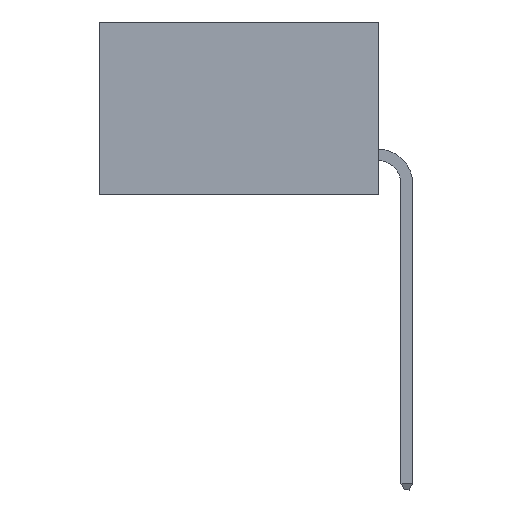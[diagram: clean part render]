
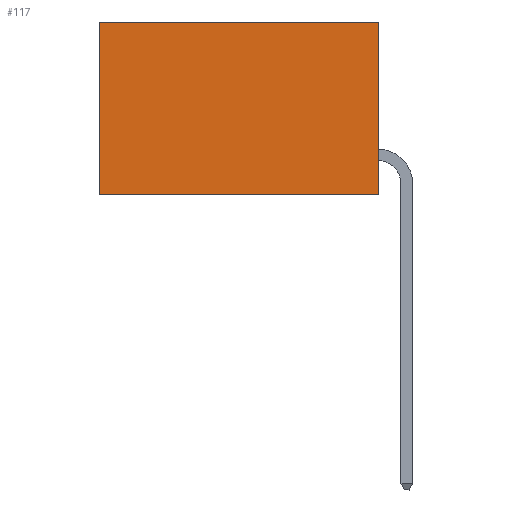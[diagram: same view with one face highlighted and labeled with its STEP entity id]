
A CAD part, left-side view. The second image highlights one B-rep face of the part: STEP entity #117.
In plain terms, the highlighted planar face has unit normal (-1, 0, 0).
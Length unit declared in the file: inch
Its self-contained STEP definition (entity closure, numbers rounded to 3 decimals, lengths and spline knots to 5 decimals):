
#40 = DIRECTION ( 'NONE',  ( 0., 0., -1. ) ) ;
#117 = ADVANCED_FACE ( 'NONE', ( #11206 ), #12971, .F. ) ;
#726 = VERTEX_POINT ( 'NONE', #10711 ) ;
#926 = DIRECTION ( 'NONE',  ( 0., 0., -1. ) ) ;
#1100 = EDGE_LOOP ( 'NONE', ( #23001, #15361, #29231, #12698 ) ) ;
#1871 = CARTESIAN_POINT ( 'NONE',  ( 0.298, 0., -0.37 ) ) ;
#2598 = VECTOR ( 'NONE', #40, 39.37008 ) ;
#3870 = EDGE_CURVE ( 'NONE', #726, #29299, #20735, .T. ) ;
#4047 = AXIS2_PLACEMENT_3D ( 'NONE', #30027, #26291, #926 ) ;
#4382 = DIRECTION ( 'NONE',  ( 0., 1., 0. ) ) ;
#4560 = CARTESIAN_POINT ( 'NONE',  ( 0.298, 0.6, 0. ) ) ;
#5540 = EDGE_CURVE ( 'NONE', #17120, #726, #23211, .T. ) ;
#6590 = LINE ( 'NONE', #20041, #15400 ) ;
#9495 = LINE ( 'NONE', #25413, #21304 ) ;
#10711 = CARTESIAN_POINT ( 'NONE',  ( 0.298, 0., -0.37 ) ) ;
#11206 = FACE_OUTER_BOUND ( 'NONE', #1100, .T. ) ;
#12698 = ORIENTED_EDGE ( 'NONE', *, *, #13210, .T. ) ;
#12971 = PLANE ( 'NONE',  #4047 ) ;
#13210 = EDGE_CURVE ( 'NONE', #17120, #13450, #9495, .T. ) ;
#13450 = VERTEX_POINT ( 'NONE', #4560 ) ;
#14958 = CARTESIAN_POINT ( 'NONE',  ( 0.298, 0., 0. ) ) ;
#15361 = ORIENTED_EDGE ( 'NONE', *, *, #3870, .F. ) ;
#15400 = VECTOR ( 'NONE', #20473, 39.37008 ) ;
#16632 = EDGE_CURVE ( 'NONE', #13450, #29299, #6590, .T. ) ;
#17120 = VERTEX_POINT ( 'NONE', #14958 ) ;
#20041 = CARTESIAN_POINT ( 'NONE',  ( 0.298, 0.6, 0. ) ) ;
#20473 = DIRECTION ( 'NONE',  ( 0., 0., -1. ) ) ;
#20735 = LINE ( 'NONE', #1871, #24355 ) ;
#21304 = VECTOR ( 'NONE', #4382, 39.37008 ) ;
#23001 = ORIENTED_EDGE ( 'NONE', *, *, #16632, .T. ) ;
#23145 = DIRECTION ( 'NONE',  ( 0., 1., 0. ) ) ;
#23211 = LINE ( 'NONE', #23463, #2598 ) ;
#23463 = CARTESIAN_POINT ( 'NONE',  ( 0.298, 0., 0. ) ) ;
#24355 = VECTOR ( 'NONE', #23145, 39.37008 ) ;
#25413 = CARTESIAN_POINT ( 'NONE',  ( 0.298, 0., 0. ) ) ;
#26291 = DIRECTION ( 'NONE',  ( 1., 0., 0. ) ) ;
#27585 = CARTESIAN_POINT ( 'NONE',  ( 0.298, 0.6, -0.37 ) ) ;
#29231 = ORIENTED_EDGE ( 'NONE', *, *, #5540, .F. ) ;
#29299 = VERTEX_POINT ( 'NONE', #27585 ) ;
#30027 = CARTESIAN_POINT ( 'NONE',  ( 0.298, 0., 0. ) ) ;
